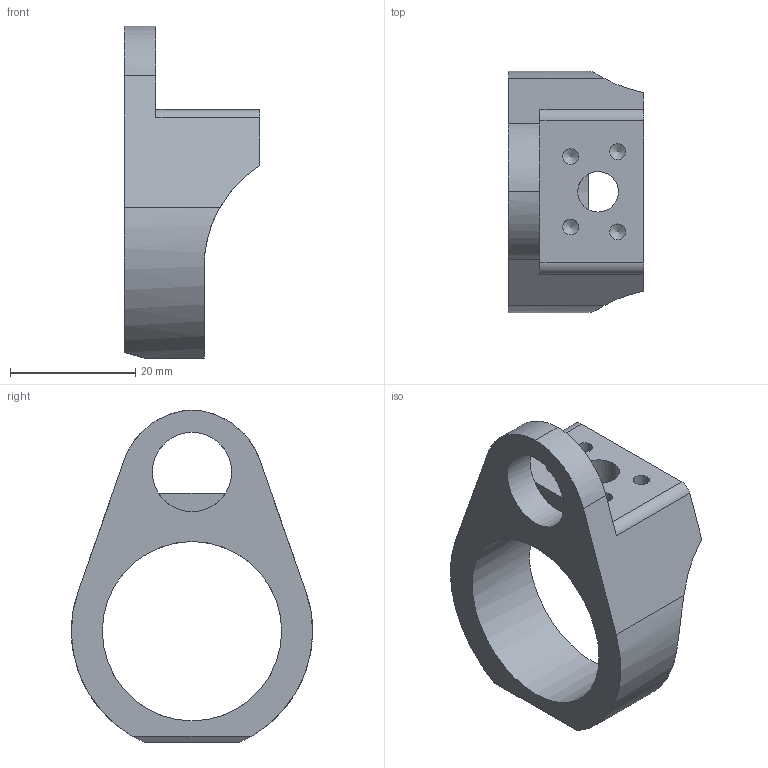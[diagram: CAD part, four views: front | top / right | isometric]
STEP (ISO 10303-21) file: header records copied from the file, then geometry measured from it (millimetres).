
FILE_DESCRIPTION(/* description */ (''),/* implementation_level */ '2;1');
FILE_NAME(/* name */ 'AR-00 Buffer Tube Adapter revA.step',/* time_stamp */ '2021-11-08T14:13:01-06:00',/* author */ (''),/* organization */ (''),/* preprocessor_version */ 'ST-DEVELOPER v18.1',/* originating_system */ 'Autodesk Translation Framework v10.10.0.1391',/* authorisation */ '');
FILE_SCHEMA (('AUTOMOTIVE_DESIGN { 1 0 10303 214 3 1 1 }'));
Length unit declared in the file: inch
Products named in the file (1): AR-00 Buffer Tube Adapter
Bounding box: 21.67 x 38.5 x 52.98 mm (x, y, z)
Volume: 11181.1 mm3; surface area: 5738.3 mm2
Topology: 1 solids, 1 shells, 29 faces, 82 edges, 53 vertices
Faces by surface type: cylinder 13, plane 10, cone 4, bspline 2
Full cylindrical faces by diameter (mm): 2.529 x4, 6.477 x1, 12.675 x1, 28.626 x1
Entity records: 1147 total; most frequent: CARTESIAN_POINT 358, ORIENTED_EDGE 156, DIRECTION 151, EDGE_CURVE 78, AXIS2_PLACEMENT_3D 56, VERTEX_POINT 53, LINE 39, VECTOR 39
